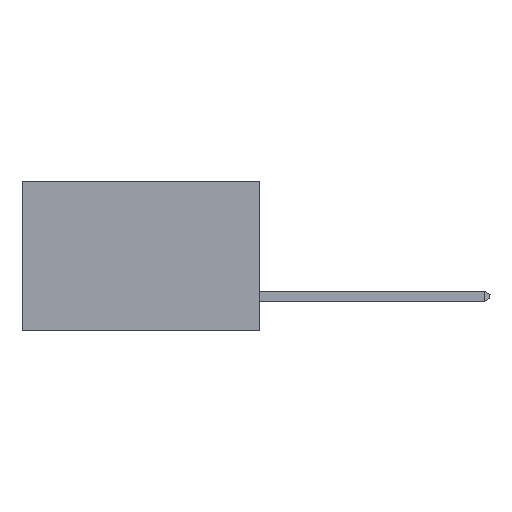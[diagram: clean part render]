
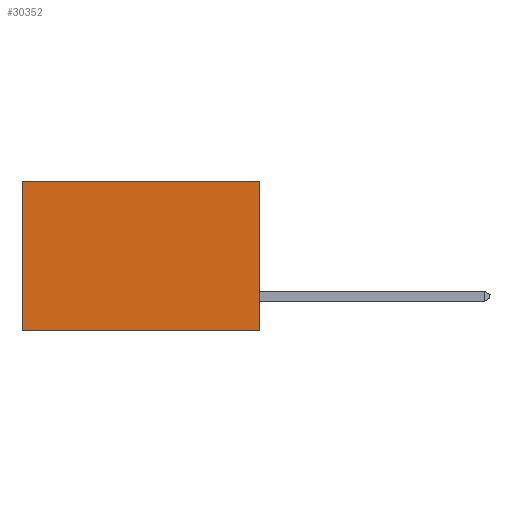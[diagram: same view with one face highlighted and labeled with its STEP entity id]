
A CAD part, left-side view. The second image highlights one B-rep face of the part: STEP entity #30352.
In plain terms, the highlighted planar face has unit normal (-1, 0, 0).
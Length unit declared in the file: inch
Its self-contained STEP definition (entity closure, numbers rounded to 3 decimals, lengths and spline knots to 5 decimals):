
#627 = DIRECTION ( 'NONE',  ( 0., 1., 0. ) ) ;
#1014 = CARTESIAN_POINT ( 'NONE',  ( 0.277, 0., -0.37 ) ) ;
#1105 = VERTEX_POINT ( 'NONE', #18112 ) ;
#1258 = CARTESIAN_POINT ( 'NONE',  ( 0.277, 0.59, -0.37 ) ) ;
#1452 = CARTESIAN_POINT ( 'NONE',  ( 0.277, 0., 0. ) ) ;
#1814 = DIRECTION ( 'NONE',  ( 0., 1., 0. ) ) ;
#2095 = DIRECTION ( 'NONE',  ( 0., 0., -1. ) ) ;
#3179 = LINE ( 'NONE', #1014, #15063 ) ;
#4539 = CARTESIAN_POINT ( 'NONE',  ( 0.277, 0.59, -0.37 ) ) ;
#5293 = EDGE_CURVE ( 'NONE', #9953, #23873, #14361, .T. ) ;
#6568 = EDGE_LOOP ( 'NONE', ( #17744, #14001, #12408, #17398 ) ) ;
#7894 = VECTOR ( 'NONE', #1814, 39.37008 ) ;
#9953 = VERTEX_POINT ( 'NONE', #1452 ) ;
#10306 = EDGE_CURVE ( 'NONE', #23873, #23840, #3179, .T. ) ;
#10969 = DIRECTION ( 'NONE',  ( 1., 0., 0. ) ) ;
#12408 = ORIENTED_EDGE ( 'NONE', *, *, #5293, .F. ) ;
#14001 = ORIENTED_EDGE ( 'NONE', *, *, #10306, .F. ) ;
#14361 = LINE ( 'NONE', #30460, #19845 ) ;
#15063 = VECTOR ( 'NONE', #627, 39.37008 ) ;
#15821 = AXIS2_PLACEMENT_3D ( 'NONE', #25012, #10969, #27386 ) ;
#17398 = ORIENTED_EDGE ( 'NONE', *, *, #17904, .T. ) ;
#17744 = ORIENTED_EDGE ( 'NONE', *, *, #19672, .T. ) ;
#17840 = PLANE ( 'NONE',  #15821 ) ;
#17904 = EDGE_CURVE ( 'NONE', #9953, #1105, #20389, .T. ) ;
#18112 = CARTESIAN_POINT ( 'NONE',  ( 0.277, 0.59, 0. ) ) ;
#19672 = EDGE_CURVE ( 'NONE', #1105, #23840, #28115, .T. ) ;
#19845 = VECTOR ( 'NONE', #27375, 39.37008 ) ;
#20389 = LINE ( 'NONE', #30092, #7894 ) ;
#22198 = FACE_OUTER_BOUND ( 'NONE', #6568, .T. ) ;
#23840 = VERTEX_POINT ( 'NONE', #1258 ) ;
#23873 = VERTEX_POINT ( 'NONE', #24918 ) ;
#24918 = CARTESIAN_POINT ( 'NONE',  ( 0.277, 0., -0.37 ) ) ;
#25012 = CARTESIAN_POINT ( 'NONE',  ( 0.277, 0., -0.37 ) ) ;
#27375 = DIRECTION ( 'NONE',  ( 0., 0., -1. ) ) ;
#27386 = DIRECTION ( 'NONE',  ( 0., 0., -1. ) ) ;
#27407 = VECTOR ( 'NONE', #2095, 39.37008 ) ;
#28115 = LINE ( 'NONE', #4539, #27407 ) ;
#30092 = CARTESIAN_POINT ( 'NONE',  ( 0.277, 0., 0. ) ) ;
#30352 = ADVANCED_FACE ( 'NONE', ( #22198 ), #17840, .F. ) ;
#30460 = CARTESIAN_POINT ( 'NONE',  ( 0.277, 0., -0.37 ) ) ;
